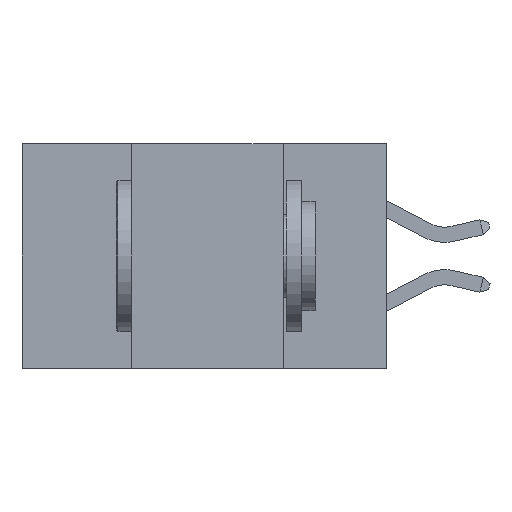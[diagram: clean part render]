
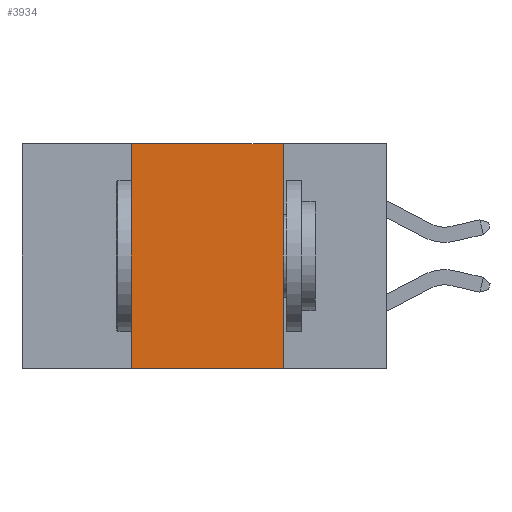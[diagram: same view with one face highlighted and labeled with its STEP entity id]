
A CAD part, left-side view. The second image highlights one B-rep face of the part: STEP entity #3934.
In plain terms, the highlighted planar face has unit normal (-1, 0, 0).
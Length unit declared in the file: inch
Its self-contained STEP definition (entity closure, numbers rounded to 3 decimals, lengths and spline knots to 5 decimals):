
#334 = CARTESIAN_POINT ( 'NONE',  ( 0., 0.6, -0.37 ) ) ;
#1402 = DIRECTION ( 'NONE',  ( 0., -1., 0. ) ) ;
#2737 = AXIS2_PLACEMENT_3D ( 'NONE', #22015, #17924, #5125 ) ;
#2960 = PLANE ( 'NONE',  #2737 ) ;
#3321 = LINE ( 'NONE', #334, #25404 ) ;
#3348 = EDGE_CURVE ( 'NONE', #16633, #19347, #17722, .T. ) ;
#3934 = ADVANCED_FACE ( 'NONE', ( #24736 ), #2960, .F. ) ;
#5002 = EDGE_CURVE ( 'NONE', #19347, #10923, #6649, .T. ) ;
#5125 = DIRECTION ( 'NONE',  ( 0., 0., -1. ) ) ;
#6341 = VECTOR ( 'NONE', #8656, 39.37008 ) ;
#6649 = LINE ( 'NONE', #19601, #6341 ) ;
#7269 = CARTESIAN_POINT ( 'NONE',  ( 0., 0.42, 0. ) ) ;
#7288 = CARTESIAN_POINT ( 'NONE',  ( 0., 0.42, -0.37 ) ) ;
#7305 = CARTESIAN_POINT ( 'NONE',  ( 0., 0.17, -0.37 ) ) ;
#8656 = DIRECTION ( 'NONE',  ( 0., 0., -1. ) ) ;
#10923 = VERTEX_POINT ( 'NONE', #7305 ) ;
#12004 = VECTOR ( 'NONE', #1402, 39.37008 ) ;
#12119 = CARTESIAN_POINT ( 'NONE',  ( 0., 0.6, 0. ) ) ;
#14863 = ORIENTED_EDGE ( 'NONE', *, *, #22839, .F. ) ;
#15018 = DIRECTION ( 'NONE',  ( 0., -1., 0. ) ) ;
#15673 = DIRECTION ( 'NONE',  ( 0., 0., 1. ) ) ;
#15933 = ORIENTED_EDGE ( 'NONE', *, *, #3348, .F. ) ;
#16633 = VERTEX_POINT ( 'NONE', #7269 ) ;
#16696 = VECTOR ( 'NONE', #15673, 39.37008 ) ;
#17173 = LINE ( 'NONE', #17661, #16696 ) ;
#17661 = CARTESIAN_POINT ( 'NONE',  ( 0., 0.42, 0. ) ) ;
#17722 = LINE ( 'NONE', #12119, #12004 ) ;
#17924 = DIRECTION ( 'NONE',  ( 1., 0., 0. ) ) ;
#17944 = CARTESIAN_POINT ( 'NONE',  ( 0., 0.17, 0. ) ) ;
#19347 = VERTEX_POINT ( 'NONE', #17944 ) ;
#19435 = VERTEX_POINT ( 'NONE', #7288 ) ;
#19601 = CARTESIAN_POINT ( 'NONE',  ( 0., 0.17, 0. ) ) ;
#21883 = EDGE_LOOP ( 'NONE', ( #27703, #15933, #14863, #24306 ) ) ;
#22015 = CARTESIAN_POINT ( 'NONE',  ( 0., 0.6, 0. ) ) ;
#22639 = EDGE_CURVE ( 'NONE', #19435, #10923, #3321, .T. ) ;
#22839 = EDGE_CURVE ( 'NONE', #19435, #16633, #17173, .T. ) ;
#24306 = ORIENTED_EDGE ( 'NONE', *, *, #22639, .T. ) ;
#24736 = FACE_OUTER_BOUND ( 'NONE', #21883, .T. ) ;
#25404 = VECTOR ( 'NONE', #15018, 39.37008 ) ;
#27703 = ORIENTED_EDGE ( 'NONE', *, *, #5002, .F. ) ;
